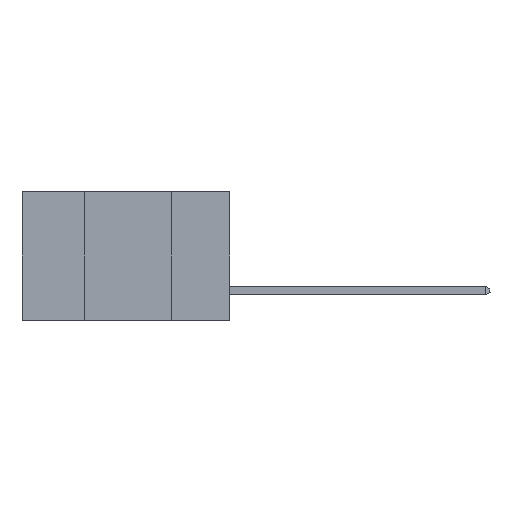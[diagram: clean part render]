
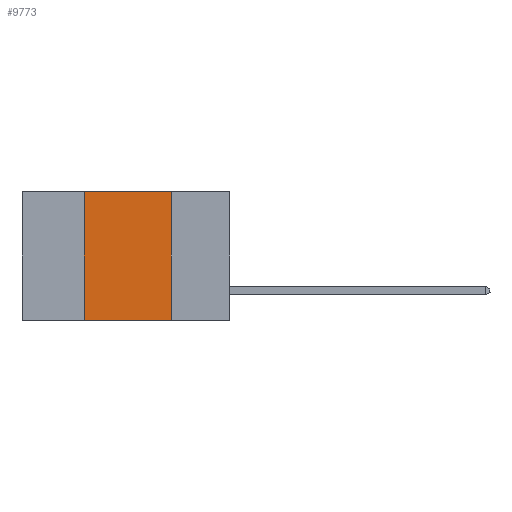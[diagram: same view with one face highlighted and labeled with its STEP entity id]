
A CAD part, left-side view. The second image highlights one B-rep face of the part: STEP entity #9773.
In plain terms, the highlighted planar face has unit normal (-1, 0, 0).
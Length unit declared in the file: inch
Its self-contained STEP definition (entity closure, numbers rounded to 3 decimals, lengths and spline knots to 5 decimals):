
#315 = VERTEX_POINT ( 'NONE', #11268 ) ;
#439 = DIRECTION ( 'NONE',  ( 0., 0., -1. ) ) ;
#837 = LINE ( 'NONE', #6347, #11572 ) ;
#1005 = CARTESIAN_POINT ( 'NONE',  ( 0., 0.6, 0. ) ) ;
#2259 = CARTESIAN_POINT ( 'NONE',  ( 0., 0.17, 0. ) ) ;
#2393 = LINE ( 'NONE', #1005, #7585 ) ;
#2594 = PLANE ( 'NONE',  #6778 ) ;
#2889 = ORIENTED_EDGE ( 'NONE', *, *, #6007, .F. ) ;
#3542 = DIRECTION ( 'NONE',  ( 0., 0., -1. ) ) ;
#3743 = EDGE_CURVE ( 'NONE', #4640, #315, #837, .T. ) ;
#3936 = CARTESIAN_POINT ( 'NONE',  ( 0., 0.42, 0. ) ) ;
#3946 = DIRECTION ( 'NONE',  ( 0., -1., 0. ) ) ;
#3956 = VECTOR ( 'NONE', #439, 39.37008 ) ;
#4059 = DIRECTION ( 'NONE',  ( 0., 0., 1. ) ) ;
#4640 = VERTEX_POINT ( 'NONE', #5232 ) ;
#5232 = CARTESIAN_POINT ( 'NONE',  ( 0., 0.42, -0.37 ) ) ;
#5257 = DIRECTION ( 'NONE',  ( 0., -1., 0. ) ) ;
#5279 = LINE ( 'NONE', #3936, #12142 ) ;
#6007 = EDGE_CURVE ( 'NONE', #6499, #10377, #2393, .T. ) ;
#6332 = CARTESIAN_POINT ( 'NONE',  ( 0., 0.42, 0. ) ) ;
#6347 = CARTESIAN_POINT ( 'NONE',  ( 0., 0.6, -0.37 ) ) ;
#6408 = CARTESIAN_POINT ( 'NONE',  ( 0., 0.6, 0. ) ) ;
#6499 = VERTEX_POINT ( 'NONE', #6332 ) ;
#6778 = AXIS2_PLACEMENT_3D ( 'NONE', #6408, #9170, #3542 ) ;
#6812 = CARTESIAN_POINT ( 'NONE',  ( 0., 0.17, 0. ) ) ;
#6920 = LINE ( 'NONE', #2259, #3956 ) ;
#7478 = FACE_OUTER_BOUND ( 'NONE', #11081, .T. ) ;
#7585 = VECTOR ( 'NONE', #3946, 39.37008 ) ;
#8087 = EDGE_CURVE ( 'NONE', #4640, #6499, #5279, .T. ) ;
#8759 = ORIENTED_EDGE ( 'NONE', *, *, #11089, .F. ) ;
#9170 = DIRECTION ( 'NONE',  ( 1., 0., 0. ) ) ;
#9773 = ADVANCED_FACE ( 'NONE', ( #7478 ), #2594, .F. ) ;
#9830 = ORIENTED_EDGE ( 'NONE', *, *, #8087, .F. ) ;
#10151 = ORIENTED_EDGE ( 'NONE', *, *, #3743, .T. ) ;
#10377 = VERTEX_POINT ( 'NONE', #6812 ) ;
#11081 = EDGE_LOOP ( 'NONE', ( #8759, #2889, #9830, #10151 ) ) ;
#11089 = EDGE_CURVE ( 'NONE', #10377, #315, #6920, .T. ) ;
#11268 = CARTESIAN_POINT ( 'NONE',  ( 0., 0.17, -0.37 ) ) ;
#11572 = VECTOR ( 'NONE', #5257, 39.37008 ) ;
#12142 = VECTOR ( 'NONE', #4059, 39.37008 ) ;
